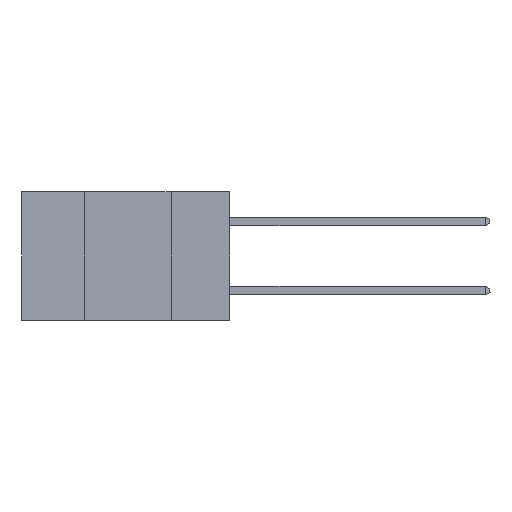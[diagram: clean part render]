
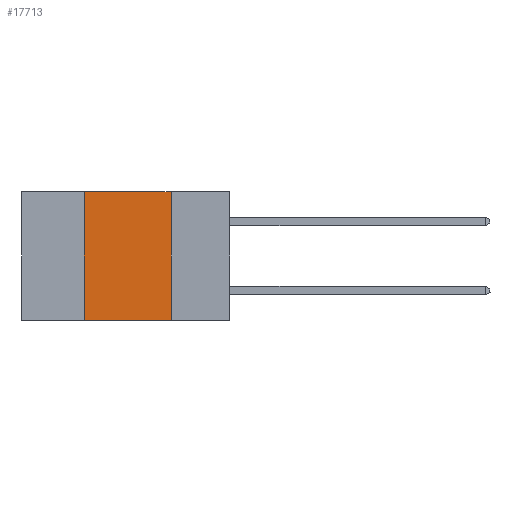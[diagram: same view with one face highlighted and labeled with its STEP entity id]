
A CAD part, left-side view. The second image highlights one B-rep face of the part: STEP entity #17713.
In plain terms, the highlighted planar face has unit normal (-1, 0, 0).
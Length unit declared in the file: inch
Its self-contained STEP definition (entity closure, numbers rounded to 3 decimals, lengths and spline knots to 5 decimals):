
#1697 = DIRECTION ( 'NONE',  ( 0., -1., 0. ) ) ;
#1808 = EDGE_CURVE ( 'NONE', #18575, #14100, #8370, .T. ) ;
#2419 = DIRECTION ( 'NONE',  ( 0., 0., -1. ) ) ;
#2609 = CARTESIAN_POINT ( 'NONE',  ( 0., 0.17, -0.37 ) ) ;
#4676 = AXIS2_PLACEMENT_3D ( 'NONE', #16535, #6913, #2419 ) ;
#6056 = EDGE_LOOP ( 'NONE', ( #23365, #7944, #26264, #17256 ) ) ;
#6634 = DIRECTION ( 'NONE',  ( 0., 0., -1. ) ) ;
#6913 = DIRECTION ( 'NONE',  ( 1., 0., 0. ) ) ;
#7152 = CARTESIAN_POINT ( 'NONE',  ( 0., 0.17, 0. ) ) ;
#7682 = VERTEX_POINT ( 'NONE', #2609 ) ;
#7944 = ORIENTED_EDGE ( 'NONE', *, *, #25664, .F. ) ;
#8061 = FACE_OUTER_BOUND ( 'NONE', #6056, .T. ) ;
#8370 = LINE ( 'NONE', #10544, #31031 ) ;
#8844 = LINE ( 'NONE', #23378, #20918 ) ;
#9857 = CARTESIAN_POINT ( 'NONE',  ( 0., 0.42, 0. ) ) ;
#10177 = CARTESIAN_POINT ( 'NONE',  ( 0., 0.6, -0.37 ) ) ;
#10544 = CARTESIAN_POINT ( 'NONE',  ( 0., 0.42, 0. ) ) ;
#12325 = EDGE_CURVE ( 'NONE', #12412, #7682, #18724, .T. ) ;
#12412 = VERTEX_POINT ( 'NONE', #7152 ) ;
#12702 = DIRECTION ( 'NONE',  ( 0., -1., 0. ) ) ;
#14020 = LINE ( 'NONE', #10177, #27574 ) ;
#14100 = VERTEX_POINT ( 'NONE', #9857 ) ;
#14936 = VECTOR ( 'NONE', #6634, 39.37008 ) ;
#16535 = CARTESIAN_POINT ( 'NONE',  ( 0., 0.6, 0. ) ) ;
#17256 = ORIENTED_EDGE ( 'NONE', *, *, #27192, .T. ) ;
#17713 = ADVANCED_FACE ( 'NONE', ( #8061 ), #28850, .F. ) ;
#18575 = VERTEX_POINT ( 'NONE', #25763 ) ;
#18724 = LINE ( 'NONE', #23197, #14936 ) ;
#20918 = VECTOR ( 'NONE', #1697, 39.37008 ) ;
#22236 = DIRECTION ( 'NONE',  ( 0., 0., 1. ) ) ;
#23197 = CARTESIAN_POINT ( 'NONE',  ( 0., 0.17, 0. ) ) ;
#23365 = ORIENTED_EDGE ( 'NONE', *, *, #12325, .F. ) ;
#23378 = CARTESIAN_POINT ( 'NONE',  ( 0., 0.6, 0. ) ) ;
#25664 = EDGE_CURVE ( 'NONE', #14100, #12412, #8844, .T. ) ;
#25763 = CARTESIAN_POINT ( 'NONE',  ( 0., 0.42, -0.37 ) ) ;
#26264 = ORIENTED_EDGE ( 'NONE', *, *, #1808, .F. ) ;
#27192 = EDGE_CURVE ( 'NONE', #18575, #7682, #14020, .T. ) ;
#27574 = VECTOR ( 'NONE', #12702, 39.37008 ) ;
#28850 = PLANE ( 'NONE',  #4676 ) ;
#31031 = VECTOR ( 'NONE', #22236, 39.37008 ) ;
